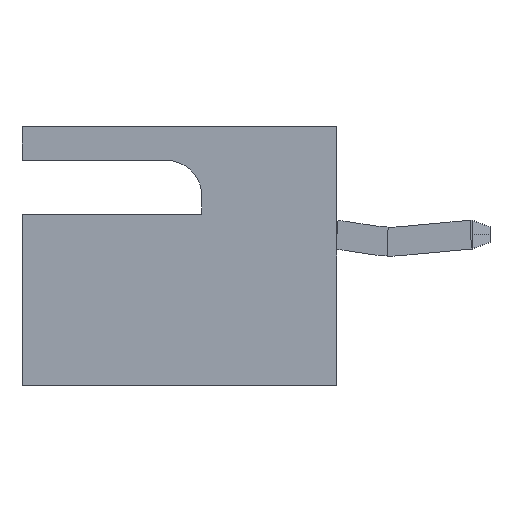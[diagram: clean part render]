
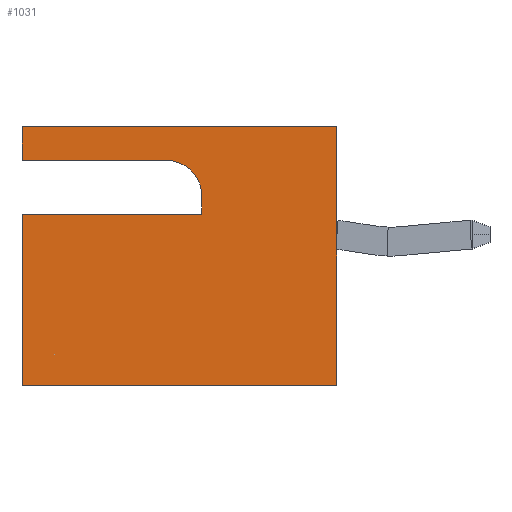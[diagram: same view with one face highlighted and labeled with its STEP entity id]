
A CAD part, left-side view. The second image highlights one B-rep face of the part: STEP entity #1031.
In plain terms, the highlighted planar face has unit normal (-1, 0, 0).
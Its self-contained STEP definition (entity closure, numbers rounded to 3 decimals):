
#28 = VECTOR ( 'NONE', #2714, 1000. ) ;
#50 = ORIENTED_EDGE ( 'NONE', *, *, #616, .F. ) ;
#143 = ORIENTED_EDGE ( 'NONE', *, *, #2200, .F. ) ;
#175 = LINE ( 'NONE', #1766, #1202 ) ;
#231 = ORIENTED_EDGE ( 'NONE', *, *, #2010, .T. ) ;
#315 = EDGE_CURVE ( 'NONE', #1647, #798, #2472, .T. ) ;
#347 = ORIENTED_EDGE ( 'NONE', *, *, #1255, .T. ) ;
#410 = CARTESIAN_POINT ( 'NONE',  ( -3.75, 7., 0.925 ) ) ;
#503 = CARTESIAN_POINT ( 'NONE',  ( -3.75, 7., 2.875 ) ) ;
#573 = DIRECTION ( 'NONE',  ( 1., 0., 0. ) ) ;
#575 = DIRECTION ( 'NONE',  ( 0., -1., 0. ) ) ;
#596 = ORIENTED_EDGE ( 'NONE', *, *, #955, .T. ) ;
#616 = EDGE_CURVE ( 'NONE', #1997, #787, #2616, .T. ) ;
#649 = DIRECTION ( 'NONE',  ( 0., 1., 0. ) ) ;
#668 = AXIS2_PLACEMENT_3D ( 'NONE', #1021, #573, #1522 ) ;
#676 = DIRECTION ( 'NONE',  ( 0., 0., -1. ) ) ;
#787 = VERTEX_POINT ( 'NONE', #796 ) ;
#791 = DIRECTION ( 'NONE',  ( 0., -1., 0. ) ) ;
#796 = CARTESIAN_POINT ( 'NONE',  ( -3.75, 0., 2.875 ) ) ;
#798 = VERTEX_POINT ( 'NONE', #2957 ) ;
#858 = VECTOR ( 'NONE', #2306, 1000. ) ;
#887 = VECTOR ( 'NONE', #791, 1000. ) ;
#930 = VERTEX_POINT ( 'NONE', #410 ) ;
#938 = EDGE_CURVE ( 'NONE', #2806, #930, #175, .T. ) ;
#955 = EDGE_CURVE ( 'NONE', #1224, #2806, #2773, .T. ) ;
#1021 = CARTESIAN_POINT ( 'NONE',  ( -3.75, 3.8, 1.325 ) ) ;
#1031 = ADVANCED_FACE ( 'NONE', ( #1670 ), #2853, .F. ) ;
#1053 = DIRECTION ( 'NONE',  ( 0., 0., 1. ) ) ;
#1081 = CARTESIAN_POINT ( 'NONE',  ( -3.75, 7., 2.125 ) ) ;
#1082 = DIRECTION ( 'NONE',  ( 0., 0., 1. ) ) ;
#1156 = ORIENTED_EDGE ( 'NONE', *, *, #315, .T. ) ;
#1174 = ORIENTED_EDGE ( 'NONE', *, *, #2005, .T. ) ;
#1202 = VECTOR ( 'NONE', #649, 1000. ) ;
#1224 = VERTEX_POINT ( 'NONE', #2536 ) ;
#1255 = EDGE_CURVE ( 'NONE', #2001, #1619, #2247, .T. ) ;
#1287 = CARTESIAN_POINT ( 'NONE',  ( -3.75, 0., -2.875 ) ) ;
#1319 = CARTESIAN_POINT ( 'NONE',  ( -3.75, 7., -2.875 ) ) ;
#1346 = CARTESIAN_POINT ( 'NONE',  ( -3.75, 3., 1.325 ) ) ;
#1522 = DIRECTION ( 'NONE',  ( 0., 0., -1. ) ) ;
#1608 = VECTOR ( 'NONE', #2510, 1000. ) ;
#1619 = VERTEX_POINT ( 'NONE', #2219 ) ;
#1647 = VERTEX_POINT ( 'NONE', #2915 ) ;
#1659 = EDGE_CURVE ( 'NONE', #1647, #930, #1757, .T. ) ;
#1670 = FACE_OUTER_BOUND ( 'NONE', #2629, .T. ) ;
#1709 = ORIENTED_EDGE ( 'NONE', *, *, #1659, .F. ) ;
#1737 = CARTESIAN_POINT ( 'NONE',  ( -3.75, 7., 2.125 ) ) ;
#1757 = LINE ( 'NONE', #1963, #28 ) ;
#1766 = CARTESIAN_POINT ( 'NONE',  ( -3.75, 7., 0.925 ) ) ;
#1907 = DIRECTION ( 'NONE',  ( 1., 0., 0. ) ) ;
#1959 = CARTESIAN_POINT ( 'NONE',  ( -3.75, 7., 2.875 ) ) ;
#1963 = CARTESIAN_POINT ( 'NONE',  ( -3.75, 7., -2.875 ) ) ;
#1997 = VERTEX_POINT ( 'NONE', #1959 ) ;
#2001 = VERTEX_POINT ( 'NONE', #1737 ) ;
#2005 = EDGE_CURVE ( 'NONE', #1619, #1224, #2712, .T. ) ;
#2010 = EDGE_CURVE ( 'NONE', #798, #787, #2478, .T. ) ;
#2112 = CARTESIAN_POINT ( 'NONE',  ( -3.75, 7., -2.875 ) ) ;
#2155 = AXIS2_PLACEMENT_3D ( 'NONE', #2112, #1907, #676 ) ;
#2200 = EDGE_CURVE ( 'NONE', #2001, #1997, #2295, .T. ) ;
#2219 = CARTESIAN_POINT ( 'NONE',  ( -3.75, 3.8, 2.125 ) ) ;
#2236 = VECTOR ( 'NONE', #1082, 1000. ) ;
#2247 = LINE ( 'NONE', #1081, #1608 ) ;
#2295 = LINE ( 'NONE', #1319, #2236 ) ;
#2306 = DIRECTION ( 'NONE',  ( 0., 0., -1. ) ) ;
#2420 = VECTOR ( 'NONE', #1053, 1000. ) ;
#2433 = VECTOR ( 'NONE', #575, 1000. ) ;
#2472 = LINE ( 'NONE', #2951, #887 ) ;
#2478 = LINE ( 'NONE', #1287, #2420 ) ;
#2510 = DIRECTION ( 'NONE',  ( 0., -1., 0. ) ) ;
#2536 = CARTESIAN_POINT ( 'NONE',  ( -3.75, 3., 1.325 ) ) ;
#2596 = ORIENTED_EDGE ( 'NONE', *, *, #938, .T. ) ;
#2616 = LINE ( 'NONE', #503, #2433 ) ;
#2629 = EDGE_LOOP ( 'NONE', ( #143, #347, #1174, #596, #2596, #1709, #1156, #231, #50 ) ) ;
#2712 = CIRCLE ( 'NONE', #668, 0.8 ) ;
#2714 = DIRECTION ( 'NONE',  ( 0., 0., 1. ) ) ;
#2773 = LINE ( 'NONE', #1346, #858 ) ;
#2806 = VERTEX_POINT ( 'NONE', #3000 ) ;
#2853 = PLANE ( 'NONE',  #2155 ) ;
#2915 = CARTESIAN_POINT ( 'NONE',  ( -3.75, 7., -2.875 ) ) ;
#2951 = CARTESIAN_POINT ( 'NONE',  ( -3.75, 7., -2.875 ) ) ;
#2957 = CARTESIAN_POINT ( 'NONE',  ( -3.75, 0., -2.875 ) ) ;
#3000 = CARTESIAN_POINT ( 'NONE',  ( -3.75, 3., 0.925 ) ) ;
